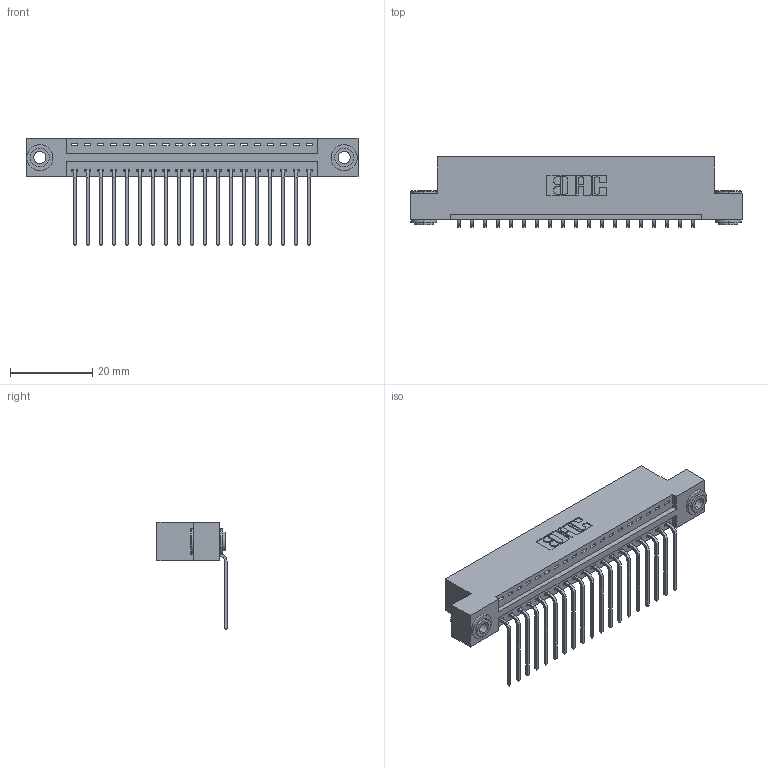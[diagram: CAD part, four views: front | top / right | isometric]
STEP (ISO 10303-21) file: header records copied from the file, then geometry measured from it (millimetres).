
FILE_DESCRIPTION (( 'STEP AP203' ), '1' );
FILE_NAME ('396-019-559-103.STEP', '2019-10-31T20:51:26', ( '' ), ( '' ), 'SwSTEP 2.0', 'SolidWorks 2016', '' );
FILE_SCHEMA (( 'CONFIG_CONTROL_DESIGN' ));
Length unit declared in the file: inch
Products named in the file (4): 396-019-559-103; 346 Part_Flush Mounting Lugs - 0.156 Dia-TH; 345-292-001_558 559 Tail - 1; 345-250-002_345-250-002-102
Assembly tree (22 placements, depth 2):
  396-019-559-103
    346 Part_Flush Mounting Lugs - 0.156 Dia-TH
    345-292-001_558 559 Tail - 1  x19
    345-250-002_345-250-002-102  x2
Bounding box: 80.9 x 17.08 x 26.16 mm (x, y, z)
Volume: 7668.1 mm3; surface area: 9932.7 mm2
Topology: 22 solids, 22 shells, 1300 faces, 3863 edges, 2546 vertices
Faces by surface type: plane 884, cylinder 408, cone 8
Entity records: 15622 total; most frequent: CARTESIAN_POINT 2664, ORIENTED_EDGE 2610, DIRECTION 2409, EDGE_CURVE 1305, LINE 1073, VECTOR 1073, VERTEX_POINT 866, AXIS2_PLACEMENT_3D 668
